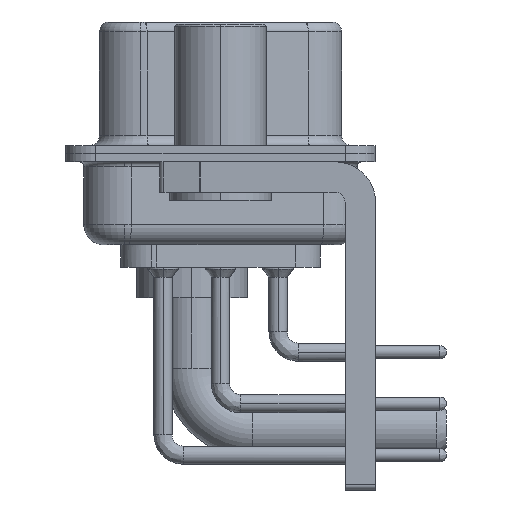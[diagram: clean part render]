
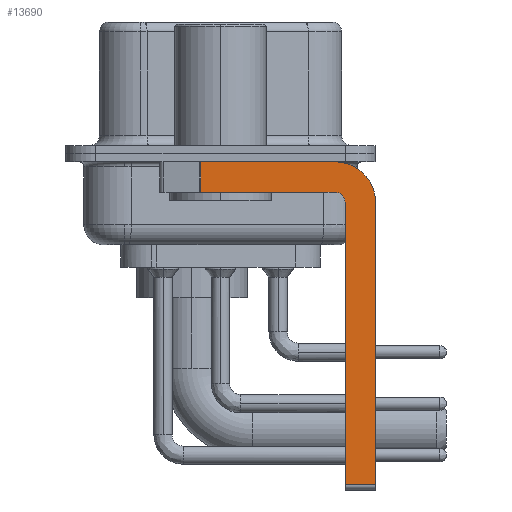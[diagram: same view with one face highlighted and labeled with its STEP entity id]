
A CAD part, left-side view. The second image highlights one B-rep face of the part: STEP entity #13690.
In plain terms, the highlighted planar face has unit normal (-1, 0, 0).
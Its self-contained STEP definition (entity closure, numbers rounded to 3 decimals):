
#336 = VERTEX_POINT ( 'NONE', #7200 ) ;
#1050 = EDGE_CURVE ( 'NONE', #23486, #22871, #3468, .T. ) ;
#1117 = VERTEX_POINT ( 'NONE', #15772 ) ;
#2695 = CARTESIAN_POINT ( 'NONE',  ( -2.9, -6.15, -16.35 ) ) ;
#3468 = LINE ( 'NONE', #24858, #34619 ) ;
#3874 = VECTOR ( 'NONE', #23672, 1000. ) ;
#4243 = VERTEX_POINT ( 'NONE', #29520 ) ;
#4692 = EDGE_CURVE ( 'NONE', #34122, #4243, #28882, .T. ) ;
#6919 = CARTESIAN_POINT ( 'NONE',  ( -2.9, 0.978, -0.4 ) ) ;
#7200 = CARTESIAN_POINT ( 'NONE',  ( -2.9, -5.65, -0.4 ) ) ;
#7374 = LINE ( 'NONE', #14800, #3874 ) ;
#7643 = CARTESIAN_POINT ( 'NONE',  ( -2.9, -5.65, -2.4 ) ) ;
#8609 = ORIENTED_EDGE ( 'NONE', *, *, #27026, .F. ) ;
#11712 = CARTESIAN_POINT ( 'NONE',  ( -2.9, -5.65, -16.35 ) ) ;
#13567 = VECTOR ( 'NONE', #31951, 1000. ) ;
#13690 = ADVANCED_FACE ( 'NONE', ( #17470 ), #30182, .F. ) ;
#14115 = CARTESIAN_POINT ( 'NONE',  ( -2.9, 0.978, -1.9 ) ) ;
#14448 = DIRECTION ( 'NONE',  ( 1., 0., 0. ) ) ;
#14800 = CARTESIAN_POINT ( 'NONE',  ( -2.9, 3., -0.4 ) ) ;
#14946 = CARTESIAN_POINT ( 'NONE',  ( -2.9, -7.65, -2.4 ) ) ;
#15190 = DIRECTION ( 'NONE',  ( -1., 0., 0. ) ) ;
#15491 = ORIENTED_EDGE ( 'NONE', *, *, #24611, .F. ) ;
#15772 = CARTESIAN_POINT ( 'NONE',  ( -2.9, -7.65, -2.4 ) ) ;
#17057 = EDGE_CURVE ( 'NONE', #35602, #22871, #37792, .T. ) ;
#17259 = CARTESIAN_POINT ( 'NONE',  ( -2.9, -5.65, -2.4 ) ) ;
#17470 = FACE_OUTER_BOUND ( 'NONE', #32672, .T. ) ;
#17596 = ORIENTED_EDGE ( 'NONE', *, *, #23535, .F. ) ;
#19236 = CIRCLE ( 'NONE', #24405, 0.5 ) ;
#19602 = CARTESIAN_POINT ( 'NONE',  ( -2.9, -5.65, -1.9 ) ) ;
#20795 = DIRECTION ( 'NONE',  ( 0., -1., 0. ) ) ;
#20911 = EDGE_CURVE ( 'NONE', #34122, #28139, #36952, .T. ) ;
#21246 = CARTESIAN_POINT ( 'NONE',  ( -2.9, -5.65, -2.4 ) ) ;
#22229 = ORIENTED_EDGE ( 'NONE', *, *, #17057, .T. ) ;
#22871 = VERTEX_POINT ( 'NONE', #14115 ) ;
#23255 = AXIS2_PLACEMENT_3D ( 'NONE', #7643, #14448, #35314 ) ;
#23324 = DIRECTION ( 'NONE',  ( 1., 0., 0. ) ) ;
#23410 = CARTESIAN_POINT ( 'NONE',  ( -2.9, -6.15, -16.6 ) ) ;
#23486 = VERTEX_POINT ( 'NONE', #19602 ) ;
#23535 = EDGE_CURVE ( 'NONE', #1117, #28139, #36538, .T. ) ;
#23672 = DIRECTION ( 'NONE',  ( 0., -1., 0. ) ) ;
#23712 = DIRECTION ( 'NONE',  ( 0., 0., -1. ) ) ;
#24405 = AXIS2_PLACEMENT_3D ( 'NONE', #21246, #15190, #27511 ) ;
#24410 = VECTOR ( 'NONE', #35934, 1000. ) ;
#24611 = EDGE_CURVE ( 'NONE', #4243, #23486, #19236, .T. ) ;
#24858 = CARTESIAN_POINT ( 'NONE',  ( -2.9, -5.65, -1.9 ) ) ;
#26627 = VECTOR ( 'NONE', #32509, 1000. ) ;
#26818 = VECTOR ( 'NONE', #20795, 1000. ) ;
#27026 = EDGE_CURVE ( 'NONE', #336, #1117, #29062, .T. ) ;
#27511 = DIRECTION ( 'NONE',  ( 0., 0., 1. ) ) ;
#27696 = ORIENTED_EDGE ( 'NONE', *, *, #20911, .T. ) ;
#27923 = ORIENTED_EDGE ( 'NONE', *, *, #4692, .F. ) ;
#28139 = VERTEX_POINT ( 'NONE', #36565 ) ;
#28709 = CARTESIAN_POINT ( 'NONE',  ( -2.9, 0.978, -1.9 ) ) ;
#28882 = LINE ( 'NONE', #23410, #26627 ) ;
#29062 = CIRCLE ( 'NONE', #23255, 2. ) ;
#29520 = CARTESIAN_POINT ( 'NONE',  ( -2.9, -6.15, -2.4 ) ) ;
#30182 = PLANE ( 'NONE',  #39593 ) ;
#31671 = ORIENTED_EDGE ( 'NONE', *, *, #38226, .F. ) ;
#31951 = DIRECTION ( 'NONE',  ( 0., 0., -1. ) ) ;
#32509 = DIRECTION ( 'NONE',  ( 0., 0., 1. ) ) ;
#32672 = EDGE_LOOP ( 'NONE', ( #31671, #22229, #34055, #15491, #27923, #27696, #17596, #8609 ) ) ;
#34055 = ORIENTED_EDGE ( 'NONE', *, *, #1050, .F. ) ;
#34122 = VERTEX_POINT ( 'NONE', #2695 ) ;
#34619 = VECTOR ( 'NONE', #37980, 1000. ) ;
#35314 = DIRECTION ( 'NONE',  ( 0., 0., -1. ) ) ;
#35602 = VERTEX_POINT ( 'NONE', #6919 ) ;
#35934 = DIRECTION ( 'NONE',  ( 0., 0., -1. ) ) ;
#36538 = LINE ( 'NONE', #14946, #24410 ) ;
#36565 = CARTESIAN_POINT ( 'NONE',  ( -2.9, -7.65, -16.35 ) ) ;
#36952 = LINE ( 'NONE', #11712, #26818 ) ;
#37792 = LINE ( 'NONE', #28709, #13567 ) ;
#37980 = DIRECTION ( 'NONE',  ( 0., 1., 0. ) ) ;
#38226 = EDGE_CURVE ( 'NONE', #35602, #336, #7374, .T. ) ;
#39593 = AXIS2_PLACEMENT_3D ( 'NONE', #17259, #23324, #23712 ) ;
